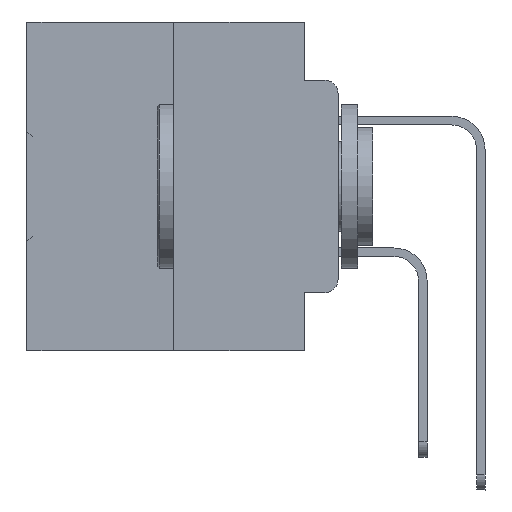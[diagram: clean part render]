
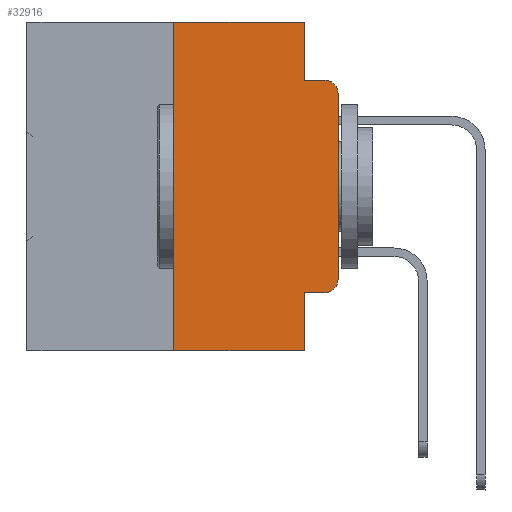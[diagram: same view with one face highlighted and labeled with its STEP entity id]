
A CAD part, left-side view. The second image highlights one B-rep face of the part: STEP entity #32916.
In plain terms, the highlighted planar face has unit normal (-1, 0, 0).
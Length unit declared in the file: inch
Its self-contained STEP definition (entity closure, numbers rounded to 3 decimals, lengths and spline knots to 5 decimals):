
#587 = CARTESIAN_POINT ( 'NONE',  ( 0., 0.051, 0. ) ) ;
#633 = DIRECTION ( 'NONE',  ( -1., 0., 0. ) ) ;
#1003 = VECTOR ( 'NONE', #3822, 39.37008 ) ;
#1649 = DIRECTION ( 'NONE',  ( 1., 0., 0. ) ) ;
#1810 = VERTEX_POINT ( 'NONE', #13084 ) ;
#2253 = CARTESIAN_POINT ( 'NONE',  ( 0., 0.02, -0.4115 ) ) ;
#3822 = DIRECTION ( 'NONE',  ( 0., -1., 0. ) ) ;
#3917 = VECTOR ( 'NONE', #32307, 39.37008 ) ;
#4715 = DIRECTION ( 'NONE',  ( 0., 0., -1. ) ) ;
#4984 = VERTEX_POINT ( 'NONE', #35156 ) ;
#5923 = EDGE_CURVE ( 'NONE', #1810, #18509, #24169, .T. ) ;
#6096 = EDGE_CURVE ( 'NONE', #11308, #25934, #13108, .T. ) ;
#7894 = DIRECTION ( 'NONE',  ( 0., 0., 1. ) ) ;
#8198 = EDGE_CURVE ( 'NONE', #33315, #25374, #23625, .T. ) ;
#8373 = CARTESIAN_POINT ( 'NONE',  ( 0., 0.473, -0.5 ) ) ;
#8639 = EDGE_CURVE ( 'NONE', #18509, #17947, #8774, .T. ) ;
#8774 = CIRCLE ( 'NONE', #35417, 0.02 ) ;
#8952 = DIRECTION ( 'NONE',  ( 0., -1., 0. ) ) ;
#9349 = DIRECTION ( 'NONE',  ( 0., 0., -1. ) ) ;
#9544 = DIRECTION ( 'NONE',  ( -1., 0., 0. ) ) ;
#9652 = EDGE_CURVE ( 'NONE', #9875, #4984, #34232, .T. ) ;
#9875 = VERTEX_POINT ( 'NONE', #587 ) ;
#10253 = LINE ( 'NONE', #33726, #15020 ) ;
#10499 = CARTESIAN_POINT ( 'NONE',  ( 0., 0., -0.3915 ) ) ;
#10610 = PLANE ( 'NONE',  #14945 ) ;
#10654 = VERTEX_POINT ( 'NONE', #26564 ) ;
#10908 = CARTESIAN_POINT ( 'NONE',  ( 0., 0.02, -0.0885 ) ) ;
#10911 = ORIENTED_EDGE ( 'NONE', *, *, #22125, .F. ) ;
#10961 = CARTESIAN_POINT ( 'NONE',  ( 0., 0.051, 0. ) ) ;
#11308 = VERTEX_POINT ( 'NONE', #34778 ) ;
#12565 = ORIENTED_EDGE ( 'NONE', *, *, #6096, .F. ) ;
#12700 = EDGE_LOOP ( 'NONE', ( #26575, #24301, #10911, #30303, #31698, #12565, #22701, #21273, #19625, #20338 ) ) ;
#12903 = CARTESIAN_POINT ( 'NONE',  ( 0., 0.02, -0.1085 ) ) ;
#13084 = CARTESIAN_POINT ( 'NONE',  ( 0., 0.051, -0.4115 ) ) ;
#13108 = LINE ( 'NONE', #34435, #25624 ) ;
#14945 = AXIS2_PLACEMENT_3D ( 'NONE', #22434, #1649, #28078 ) ;
#15020 = VECTOR ( 'NONE', #7894, 39.37008 ) ;
#15878 = VECTOR ( 'NONE', #24553, 39.37008 ) ;
#17459 = AXIS2_PLACEMENT_3D ( 'NONE', #12903, #633, #21051 ) ;
#17847 = EDGE_CURVE ( 'NONE', #1810, #10654, #30103, .T. ) ;
#17947 = VERTEX_POINT ( 'NONE', #10499 ) ;
#18509 = VERTEX_POINT ( 'NONE', #2253 ) ;
#19058 = EDGE_CURVE ( 'NONE', #25934, #9875, #37742, .T. ) ;
#19625 = ORIENTED_EDGE ( 'NONE', *, *, #5923, .T. ) ;
#20338 = ORIENTED_EDGE ( 'NONE', *, *, #8639, .T. ) ;
#21051 = DIRECTION ( 'NONE',  ( 0., 0., -1. ) ) ;
#21179 = CARTESIAN_POINT ( 'NONE',  ( 0., 0.051, 0. ) ) ;
#21273 = ORIENTED_EDGE ( 'NONE', *, *, #17847, .F. ) ;
#21640 = CARTESIAN_POINT ( 'NONE',  ( 0., 0.051, -0.4115 ) ) ;
#22125 = EDGE_CURVE ( 'NONE', #4984, #25374, #24996, .T. ) ;
#22410 = VECTOR ( 'NONE', #8952, 39.37008 ) ;
#22434 = CARTESIAN_POINT ( 'NONE',  ( 0., 0.473, 0. ) ) ;
#22691 = CARTESIAN_POINT ( 'NONE',  ( 0., 0.25, 0. ) ) ;
#22701 = ORIENTED_EDGE ( 'NONE', *, *, #28595, .T. ) ;
#23625 = CIRCLE ( 'NONE', #17459, 0.02 ) ;
#23915 = CARTESIAN_POINT ( 'NONE',  ( 0., 0.02, -0.3915 ) ) ;
#24169 = LINE ( 'NONE', #21640, #15878 ) ;
#24301 = ORIENTED_EDGE ( 'NONE', *, *, #8198, .T. ) ;
#24553 = DIRECTION ( 'NONE',  ( 0., -1., 0. ) ) ;
#24635 = VECTOR ( 'NONE', #33586, 39.37008 ) ;
#24800 = CARTESIAN_POINT ( 'NONE',  ( 0., 0.051, -0.0885 ) ) ;
#24996 = LINE ( 'NONE', #24800, #1003 ) ;
#25374 = VERTEX_POINT ( 'NONE', #10908 ) ;
#25624 = VECTOR ( 'NONE', #30940, 39.37008 ) ;
#25934 = VERTEX_POINT ( 'NONE', #22691 ) ;
#26564 = CARTESIAN_POINT ( 'NONE',  ( 0., 0.051, -0.5 ) ) ;
#26575 = ORIENTED_EDGE ( 'NONE', *, *, #34291, .T. ) ;
#28078 = DIRECTION ( 'NONE',  ( 0., 0., -1. ) ) ;
#28595 = EDGE_CURVE ( 'NONE', #11308, #10654, #35538, .T. ) ;
#30103 = LINE ( 'NONE', #21179, #24635 ) ;
#30303 = ORIENTED_EDGE ( 'NONE', *, *, #9652, .F. ) ;
#30940 = DIRECTION ( 'NONE',  ( 0., 0., 1. ) ) ;
#31698 = ORIENTED_EDGE ( 'NONE', *, *, #19058, .F. ) ;
#32307 = DIRECTION ( 'NONE',  ( 0., -1., 0. ) ) ;
#32916 = ADVANCED_FACE ( 'NONE', ( #33899 ), #10610, .F. ) ;
#33315 = VERTEX_POINT ( 'NONE', #35622 ) ;
#33586 = DIRECTION ( 'NONE',  ( 0., 0., -1. ) ) ;
#33726 = CARTESIAN_POINT ( 'NONE',  ( 0., 0., 0. ) ) ;
#33899 = FACE_OUTER_BOUND ( 'NONE', #12700, .T. ) ;
#34232 = LINE ( 'NONE', #10961, #36082 ) ;
#34291 = EDGE_CURVE ( 'NONE', #17947, #33315, #10253, .T. ) ;
#34435 = CARTESIAN_POINT ( 'NONE',  ( 0., 0.25, 0. ) ) ;
#34778 = CARTESIAN_POINT ( 'NONE',  ( 0., 0.25, -0.5 ) ) ;
#35156 = CARTESIAN_POINT ( 'NONE',  ( 0., 0.051, -0.0885 ) ) ;
#35404 = CARTESIAN_POINT ( 'NONE',  ( 0., 0.473, 0. ) ) ;
#35417 = AXIS2_PLACEMENT_3D ( 'NONE', #23915, #9544, #9349 ) ;
#35538 = LINE ( 'NONE', #8373, #22410 ) ;
#35622 = CARTESIAN_POINT ( 'NONE',  ( 0., 0., -0.1085 ) ) ;
#36082 = VECTOR ( 'NONE', #4715, 39.37008 ) ;
#37742 = LINE ( 'NONE', #35404, #3917 ) ;
